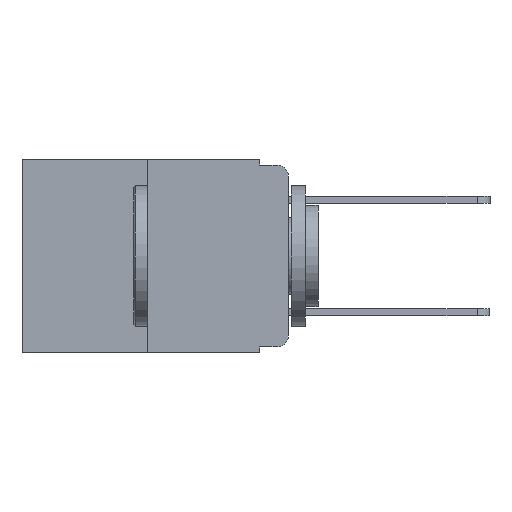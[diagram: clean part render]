
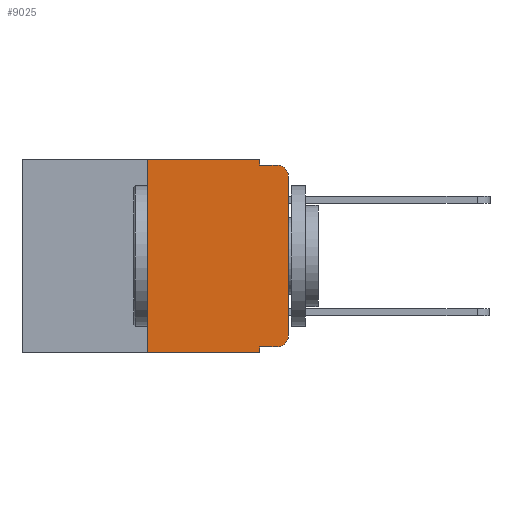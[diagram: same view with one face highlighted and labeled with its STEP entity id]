
A CAD part, left-side view. The second image highlights one B-rep face of the part: STEP entity #9025.
In plain terms, the highlighted planar face has unit normal (-1, 0, 0).
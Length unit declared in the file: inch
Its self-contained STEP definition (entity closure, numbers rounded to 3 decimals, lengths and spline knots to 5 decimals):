
#201 = CARTESIAN_POINT ( 'NONE',  ( 0., 0.25, 0. ) ) ;
#276 = CARTESIAN_POINT ( 'NONE',  ( 0., 0.02, -0.03 ) ) ;
#340 = CARTESIAN_POINT ( 'NONE',  ( 0., 0.051, 0. ) ) ;
#376 = CARTESIAN_POINT ( 'NONE',  ( 0., 0.02, -0.313 ) ) ;
#435 = ORIENTED_EDGE ( 'NONE', *, *, #6448, .F. ) ;
#534 = AXIS2_PLACEMENT_3D ( 'NONE', #2604, #7546, #2646 ) ;
#546 = VECTOR ( 'NONE', #7039, 39.37008 ) ;
#555 = DIRECTION ( 'NONE',  ( 0., -1., 0. ) ) ;
#650 = ORIENTED_EDGE ( 'NONE', *, *, #3172, .F. ) ;
#860 = ORIENTED_EDGE ( 'NONE', *, *, #5985, .T. ) ;
#985 = VECTOR ( 'NONE', #8686, 39.37008 ) ;
#1155 = DIRECTION ( 'NONE',  ( 0., 0., -1. ) ) ;
#1217 = DIRECTION ( 'NONE',  ( 0., -1., 0. ) ) ;
#1248 = DIRECTION ( 'NONE',  ( 0., 0., -1. ) ) ;
#1651 = CARTESIAN_POINT ( 'NONE',  ( 0., 0.051, -0.333 ) ) ;
#1712 = PLANE ( 'NONE',  #534 ) ;
#1914 = CARTESIAN_POINT ( 'NONE',  ( 0., 0.02, -0.333 ) ) ;
#1974 = LINE ( 'NONE', #10421, #10214 ) ;
#2347 = VERTEX_POINT ( 'NONE', #1651 ) ;
#2419 = CIRCLE ( 'NONE', #3158, 0.02 ) ;
#2464 = CARTESIAN_POINT ( 'NONE',  ( 0., 0., 0. ) ) ;
#2478 = LINE ( 'NONE', #340, #3950 ) ;
#2479 = VERTEX_POINT ( 'NONE', #201 ) ;
#2572 = VECTOR ( 'NONE', #1217, 39.37008 ) ;
#2604 = CARTESIAN_POINT ( 'NONE',  ( 0., 0.473, 0. ) ) ;
#2646 = DIRECTION ( 'NONE',  ( 0., 0., -1. ) ) ;
#2744 = VERTEX_POINT ( 'NONE', #10471 ) ;
#3053 = EDGE_CURVE ( 'NONE', #2347, #9896, #2478, .T. ) ;
#3158 = AXIS2_PLACEMENT_3D ( 'NONE', #376, #6300, #1248 ) ;
#3172 = EDGE_CURVE ( 'NONE', #2744, #6976, #5144, .T. ) ;
#3451 = CARTESIAN_POINT ( 'NONE',  ( 0., 0., -0.313 ) ) ;
#3718 = FACE_OUTER_BOUND ( 'NONE', #4208, .T. ) ;
#3763 = VERTEX_POINT ( 'NONE', #3886 ) ;
#3798 = ORIENTED_EDGE ( 'NONE', *, *, #8972, .F. ) ;
#3840 = LINE ( 'NONE', #6168, #7855 ) ;
#3842 = ORIENTED_EDGE ( 'NONE', *, *, #3053, .F. ) ;
#3886 = CARTESIAN_POINT ( 'NONE',  ( 0., 0.25, -0.343 ) ) ;
#3950 = VECTOR ( 'NONE', #7015, 39.37008 ) ;
#4002 = LINE ( 'NONE', #5653, #6193 ) ;
#4208 = EDGE_LOOP ( 'NONE', ( #860, #5762, #435, #650, #8802, #3798, #6118, #3842, #7325, #5311 ) ) ;
#4252 = DIRECTION ( 'NONE',  ( 0., 0., 1. ) ) ;
#4452 = CARTESIAN_POINT ( 'NONE',  ( 0., 0.051, -0.01 ) ) ;
#4846 = EDGE_CURVE ( 'NONE', #3763, #9896, #5261, .T. ) ;
#4852 = LINE ( 'NONE', #7838, #2572 ) ;
#5144 = LINE ( 'NONE', #6397, #7260 ) ;
#5261 = LINE ( 'NONE', #9963, #985 ) ;
#5311 = ORIENTED_EDGE ( 'NONE', *, *, #7123, .T. ) ;
#5595 = CARTESIAN_POINT ( 'NONE',  ( 0., 0., -0.03 ) ) ;
#5653 = CARTESIAN_POINT ( 'NONE',  ( 0., 0.473, 0. ) ) ;
#5708 = CARTESIAN_POINT ( 'NONE',  ( 0., 0.051, -0.343 ) ) ;
#5762 = ORIENTED_EDGE ( 'NONE', *, *, #9628, .T. ) ;
#5774 = CIRCLE ( 'NONE', #8404, 0.02 ) ;
#5985 = EDGE_CURVE ( 'NONE', #6214, #7730, #7237, .T. ) ;
#6118 = ORIENTED_EDGE ( 'NONE', *, *, #4846, .T. ) ;
#6168 = CARTESIAN_POINT ( 'NONE',  ( 0., 0.051, -0.333 ) ) ;
#6193 = VECTOR ( 'NONE', #555, 39.37008 ) ;
#6209 = DIRECTION ( 'NONE',  ( -1., 0., 0. ) ) ;
#6214 = VERTEX_POINT ( 'NONE', #3451 ) ;
#6300 = DIRECTION ( 'NONE',  ( -1., 0., 0. ) ) ;
#6397 = CARTESIAN_POINT ( 'NONE',  ( 0., 0.051, 0. ) ) ;
#6448 = EDGE_CURVE ( 'NONE', #6976, #9115, #4852, .T. ) ;
#6953 = DIRECTION ( 'NONE',  ( 0., 0., -1. ) ) ;
#6976 = VERTEX_POINT ( 'NONE', #4452 ) ;
#6977 = DIRECTION ( 'NONE',  ( 0., -1., 0. ) ) ;
#7015 = DIRECTION ( 'NONE',  ( 0., 0., -1. ) ) ;
#7039 = DIRECTION ( 'NONE',  ( 0., 0., 1. ) ) ;
#7123 = EDGE_CURVE ( 'NONE', #8676, #6214, #2419, .T. ) ;
#7237 = LINE ( 'NONE', #2464, #546 ) ;
#7260 = VECTOR ( 'NONE', #6953, 39.37008 ) ;
#7325 = ORIENTED_EDGE ( 'NONE', *, *, #9619, .T. ) ;
#7546 = DIRECTION ( 'NONE',  ( 1., 0., 0. ) ) ;
#7730 = VERTEX_POINT ( 'NONE', #5595 ) ;
#7749 = EDGE_CURVE ( 'NONE', #2479, #2744, #4002, .T. ) ;
#7838 = CARTESIAN_POINT ( 'NONE',  ( 0., 0.051, -0.01 ) ) ;
#7855 = VECTOR ( 'NONE', #6977, 39.37008 ) ;
#8404 = AXIS2_PLACEMENT_3D ( 'NONE', #276, #6209, #1155 ) ;
#8406 = CARTESIAN_POINT ( 'NONE',  ( 0., 0.02, -0.01 ) ) ;
#8676 = VERTEX_POINT ( 'NONE', #1914 ) ;
#8686 = DIRECTION ( 'NONE',  ( 0., -1., 0. ) ) ;
#8802 = ORIENTED_EDGE ( 'NONE', *, *, #7749, .F. ) ;
#8972 = EDGE_CURVE ( 'NONE', #3763, #2479, #1974, .T. ) ;
#9025 = ADVANCED_FACE ( 'NONE', ( #3718 ), #1712, .F. ) ;
#9115 = VERTEX_POINT ( 'NONE', #8406 ) ;
#9619 = EDGE_CURVE ( 'NONE', #2347, #8676, #3840, .T. ) ;
#9628 = EDGE_CURVE ( 'NONE', #7730, #9115, #5774, .T. ) ;
#9896 = VERTEX_POINT ( 'NONE', #5708 ) ;
#9963 = CARTESIAN_POINT ( 'NONE',  ( 0., 0.473, -0.343 ) ) ;
#10214 = VECTOR ( 'NONE', #4252, 39.37008 ) ;
#10421 = CARTESIAN_POINT ( 'NONE',  ( 0., 0.25, 0. ) ) ;
#10471 = CARTESIAN_POINT ( 'NONE',  ( 0., 0.051, 0. ) ) ;
